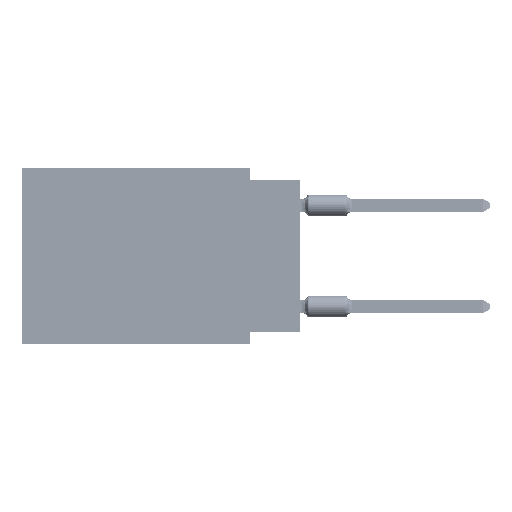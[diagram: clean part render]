
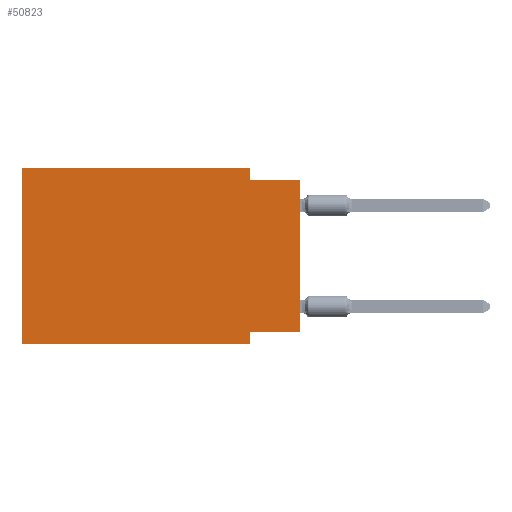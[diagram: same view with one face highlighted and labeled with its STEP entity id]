
A CAD part, left-side view. The second image highlights one B-rep face of the part: STEP entity #50823.
In plain terms, the highlighted planar face has unit normal (-1, 0, 0).
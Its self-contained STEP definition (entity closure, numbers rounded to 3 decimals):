
#1162 = CARTESIAN_POINT ( 'NONE',  ( 0., 13.97, 0. ) ) ;
#1618 = DIRECTION ( 'NONE',  ( 0., 0., -1. ) ) ;
#2724 = LINE ( 'NONE', #44079, #34459 ) ;
#4554 = CARTESIAN_POINT ( 'NONE',  ( 0., 0., -0.635 ) ) ;
#7719 = EDGE_CURVE ( 'NONE', #63672, #81472, #71573, .T. ) ;
#8679 = CARTESIAN_POINT ( 'NONE',  ( 0., 2.54, -8.89 ) ) ;
#9410 = CARTESIAN_POINT ( 'NONE',  ( 0., 13.97, -8.89 ) ) ;
#10124 = VECTOR ( 'NONE', #10408, 1000. ) ;
#10408 = DIRECTION ( 'NONE',  ( 0., -1., 0. ) ) ;
#13996 = DIRECTION ( 'NONE',  ( 0., 0., 1. ) ) ;
#15397 = DIRECTION ( 'NONE',  ( 1., 0., 0. ) ) ;
#15604 = LINE ( 'NONE', #57827, #76987 ) ;
#18460 = EDGE_CURVE ( 'NONE', #29038, #74199, #47528, .T. ) ;
#18651 = DIRECTION ( 'NONE',  ( 0., 0., -1. ) ) ;
#18860 = CARTESIAN_POINT ( 'NONE',  ( 0., 2.54, -8.255 ) ) ;
#19267 = VECTOR ( 'NONE', #36695, 1000. ) ;
#20007 = CARTESIAN_POINT ( 'NONE',  ( 0., 0., -8.255 ) ) ;
#23058 = VECTOR ( 'NONE', #45057, 1000. ) ;
#27387 = ORIENTED_EDGE ( 'NONE', *, *, #67023, .T. ) ;
#28061 = CARTESIAN_POINT ( 'NONE',  ( 0., 2.54, -8.89 ) ) ;
#29038 = VERTEX_POINT ( 'NONE', #9410 ) ;
#30306 = DIRECTION ( 'NONE',  ( 0., -1., 0. ) ) ;
#30634 = VECTOR ( 'NONE', #18651, 1000. ) ;
#32109 = ORIENTED_EDGE ( 'NONE', *, *, #44272, .F. ) ;
#32890 = CARTESIAN_POINT ( 'NONE',  ( 0., 2.54, 0. ) ) ;
#34459 = VECTOR ( 'NONE', #44515, 1000. ) ;
#36695 = DIRECTION ( 'NONE',  ( 0., 0., -1. ) ) ;
#38592 = ORIENTED_EDGE ( 'NONE', *, *, #49215, .F. ) ;
#38624 = LINE ( 'NONE', #86855, #23058 ) ;
#40094 = CARTESIAN_POINT ( 'NONE',  ( 0., 2.54, 0. ) ) ;
#41005 = ORIENTED_EDGE ( 'NONE', *, *, #18460, .F. ) ;
#43102 = EDGE_LOOP ( 'NONE', ( #27387, #32109, #80998, #38592, #41005, #66016, #62522, #72582 ) ) ;
#44079 = CARTESIAN_POINT ( 'NONE',  ( 0., 13.97, -8.89 ) ) ;
#44272 = EDGE_CURVE ( 'NONE', #54374, #55785, #15604, .T. ) ;
#44515 = DIRECTION ( 'NONE',  ( 0., -1., 0. ) ) ;
#44963 = CARTESIAN_POINT ( 'NONE',  ( 0., 2.54, -0.635 ) ) ;
#45057 = DIRECTION ( 'NONE',  ( 0., 0., 1. ) ) ;
#45301 = CARTESIAN_POINT ( 'NONE',  ( 0., 13.97, 0. ) ) ;
#45523 = EDGE_CURVE ( 'NONE', #29038, #81472, #2724, .T. ) ;
#47528 = LINE ( 'NONE', #76890, #59494 ) ;
#49215 = EDGE_CURVE ( 'NONE', #74199, #83865, #67330, .T. ) ;
#50823 = ADVANCED_FACE ( 'NONE', ( #64526 ), #64076, .F. ) ;
#54374 = VERTEX_POINT ( 'NONE', #44963 ) ;
#55785 = VERTEX_POINT ( 'NONE', #4554 ) ;
#56525 = EDGE_CURVE ( 'NONE', #84963, #63672, #82908, .T. ) ;
#57287 = LINE ( 'NONE', #32890, #30634 ) ;
#57827 = CARTESIAN_POINT ( 'NONE',  ( 0., 0., -0.635 ) ) ;
#59494 = VECTOR ( 'NONE', #13996, 1000. ) ;
#62522 = ORIENTED_EDGE ( 'NONE', *, *, #7719, .F. ) ;
#63672 = VERTEX_POINT ( 'NONE', #18860 ) ;
#64076 = PLANE ( 'NONE',  #83702 ) ;
#64526 = FACE_OUTER_BOUND ( 'NONE', #43102, .T. ) ;
#66016 = ORIENTED_EDGE ( 'NONE', *, *, #45523, .T. ) ;
#67023 = EDGE_CURVE ( 'NONE', #84963, #55785, #38624, .T. ) ;
#67330 = LINE ( 'NONE', #45301, #10124 ) ;
#70600 = CARTESIAN_POINT ( 'NONE',  ( 0., 0., -8.255 ) ) ;
#71573 = LINE ( 'NONE', #8679, #19267 ) ;
#72582 = ORIENTED_EDGE ( 'NONE', *, *, #56525, .F. ) ;
#74199 = VERTEX_POINT ( 'NONE', #86712 ) ;
#76014 = DIRECTION ( 'NONE',  ( 0., 1., 0. ) ) ;
#76890 = CARTESIAN_POINT ( 'NONE',  ( 0., 13.97, 0. ) ) ;
#76987 = VECTOR ( 'NONE', #30306, 1000. ) ;
#77488 = EDGE_CURVE ( 'NONE', #83865, #54374, #57287, .T. ) ;
#80649 = VECTOR ( 'NONE', #76014, 1000. ) ;
#80998 = ORIENTED_EDGE ( 'NONE', *, *, #77488, .F. ) ;
#81472 = VERTEX_POINT ( 'NONE', #28061 ) ;
#82908 = LINE ( 'NONE', #20007, #80649 ) ;
#83702 = AXIS2_PLACEMENT_3D ( 'NONE', #1162, #15397, #1618 ) ;
#83865 = VERTEX_POINT ( 'NONE', #40094 ) ;
#84963 = VERTEX_POINT ( 'NONE', #70600 ) ;
#86712 = CARTESIAN_POINT ( 'NONE',  ( 0., 13.97, 0. ) ) ;
#86855 = CARTESIAN_POINT ( 'NONE',  ( 0., 0., 0. ) ) ;
